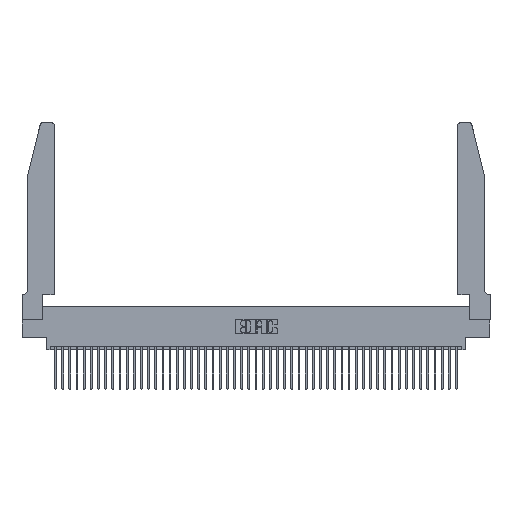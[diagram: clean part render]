
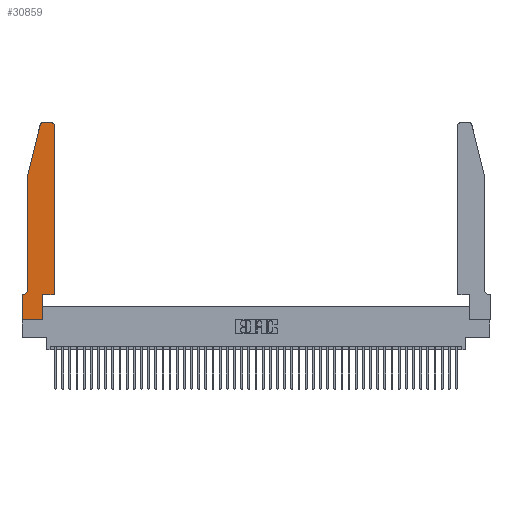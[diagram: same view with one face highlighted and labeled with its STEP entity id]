
A CAD part, top view. The second image highlights one B-rep face of the part: STEP entity #30859.
In plain terms, the highlighted planar face has unit normal (0, 0, 1).
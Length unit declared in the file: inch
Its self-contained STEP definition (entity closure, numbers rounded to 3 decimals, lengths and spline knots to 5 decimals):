
#106 = DIRECTION ( 'NONE',  ( -0.239, -0.971, 0. ) ) ;
#326 = PLANE ( 'NONE',  #36284 ) ;
#693 = LINE ( 'NONE', #32743, #38862 ) ;
#1803 = CARTESIAN_POINT ( 'NONE',  ( 0.0755, 0.42, 0.37 ) ) ;
#2309 = ORIENTED_EDGE ( 'NONE', *, *, #7691, .T. ) ;
#3021 = DIRECTION ( 'NONE',  ( 1., 0., 0. ) ) ;
#4011 = EDGE_CURVE ( 'NONE', #29170, #10294, #20883, .T. ) ;
#4513 = AXIS2_PLACEMENT_3D ( 'NONE', #14572, #40284, #18308 ) ;
#4739 = VERTEX_POINT ( 'NONE', #24880 ) ;
#4830 = EDGE_CURVE ( 'NONE', #10294, #25351, #20247, .T. ) ;
#5912 = VERTEX_POINT ( 'NONE', #9703 ) ;
#6037 = CARTESIAN_POINT ( 'NONE',  ( 0., 0., 0.37 ) ) ;
#6311 = VERTEX_POINT ( 'NONE', #16359 ) ;
#6800 = EDGE_CURVE ( 'NONE', #5912, #36614, #37261, .T. ) ;
#7691 = EDGE_CURVE ( 'NONE', #46700, #10394, #33453, .T. ) ;
#7784 = DIRECTION ( 'NONE',  ( 0., 0., 1. ) ) ;
#8949 = VECTOR ( 'NONE', #31866, 39.37008 ) ;
#9164 = EDGE_CURVE ( 'NONE', #25351, #6311, #40741, .T. ) ;
#9679 = ORIENTED_EDGE ( 'NONE', *, *, #36861, .T. ) ;
#9703 = CARTESIAN_POINT ( 'NONE',  ( 0., 0.35, 0.37 ) ) ;
#9863 = DIRECTION ( 'NONE',  ( 1., 0., 0. ) ) ;
#10294 = VERTEX_POINT ( 'NONE', #19686 ) ;
#10343 = CARTESIAN_POINT ( 'NONE',  ( 0.0755, 0.35, 0.37 ) ) ;
#10394 = VERTEX_POINT ( 'NONE', #12528 ) ;
#10613 = CARTESIAN_POINT ( 'NONE',  ( 0.2865, 0.35, 0.37 ) ) ;
#11379 = VECTOR ( 'NONE', #12833, 39.37008 ) ;
#12073 = VECTOR ( 'NONE', #32721, 39.37008 ) ;
#12437 = VECTOR ( 'NONE', #9863, 39.37008 ) ;
#12528 = CARTESIAN_POINT ( 'NONE',  ( 0.0755, 2., 0.37 ) ) ;
#12833 = DIRECTION ( 'NONE',  ( -1., 0., 0. ) ) ;
#12932 = AXIS2_PLACEMENT_3D ( 'NONE', #40103, #18118, #43701 ) ;
#13871 = ORIENTED_EDGE ( 'NONE', *, *, #18072, .T. ) ;
#14120 = DIRECTION ( 'NONE',  ( -1., 0., 0. ) ) ;
#14572 = CARTESIAN_POINT ( 'NONE',  ( 0.0055, 0.42, 0.37 ) ) ;
#14804 = CARTESIAN_POINT ( 'NONE',  ( 0.4505, 0.35, 0.37 ) ) ;
#16359 = CARTESIAN_POINT ( 'NONE',  ( 0.284, 2.75, 0.37 ) ) ;
#16466 = ORIENTED_EDGE ( 'NONE', *, *, #4830, .T. ) ;
#17728 = VECTOR ( 'NONE', #14120, 39.37008 ) ;
#18072 = EDGE_CURVE ( 'NONE', #18922, #29108, #40275, .T. ) ;
#18118 = DIRECTION ( 'NONE',  ( 0., 0., 1. ) ) ;
#18139 = DIRECTION ( 'NONE',  ( 0., -1., 0. ) ) ;
#18308 = DIRECTION ( 'NONE',  ( -1., 0., 0. ) ) ;
#18481 = ORIENTED_EDGE ( 'NONE', *, *, #43101, .T. ) ;
#18615 = VECTOR ( 'NONE', #3021, 39.37008 ) ;
#18922 = VERTEX_POINT ( 'NONE', #33369 ) ;
#19596 = CARTESIAN_POINT ( 'NONE',  ( 0.284, 2.72, 0.37 ) ) ;
#19686 = CARTESIAN_POINT ( 'NONE',  ( 0.4505, 2.72, 0.37 ) ) ;
#20041 = ORIENTED_EDGE ( 'NONE', *, *, #21690, .T. ) ;
#20247 = CIRCLE ( 'NONE', #12932, 0.03 ) ;
#20604 = CARTESIAN_POINT ( 'NONE',  ( 0.25487, 2.72718, 0.37 ) ) ;
#20883 = LINE ( 'NONE', #20950, #39261 ) ;
#20950 = CARTESIAN_POINT ( 'NONE',  ( 0.4505, 0.35, 0.37 ) ) ;
#21690 = EDGE_CURVE ( 'NONE', #36614, #18922, #23450, .T. ) ;
#22193 = CARTESIAN_POINT ( 'NONE',  ( 0.0755, 2., 0.37 ) ) ;
#22351 = FACE_OUTER_BOUND ( 'NONE', #24355, .T. ) ;
#22957 = ORIENTED_EDGE ( 'NONE', *, *, #46926, .T. ) ;
#23303 = DIRECTION ( 'NONE',  ( 1., 0., 0. ) ) ;
#23450 = LINE ( 'NONE', #28476, #12437 ) ;
#23678 = ORIENTED_EDGE ( 'NONE', *, *, #31571, .T. ) ;
#23704 = VECTOR ( 'NONE', #106, 39.37008 ) ;
#24355 = EDGE_LOOP ( 'NONE', ( #29853, #23678, #2309, #9679, #22957, #18481, #30250, #20041, #13871, #29082, #36806, #16466 ) ) ;
#24656 = CIRCLE ( 'NONE', #4513, 0.07 ) ;
#24880 = CARTESIAN_POINT ( 'NONE',  ( 0.0055, 0.35, 0.37 ) ) ;
#25211 = CARTESIAN_POINT ( 'NONE',  ( 0.4505, 0.35, 0.37 ) ) ;
#25351 = VERTEX_POINT ( 'NONE', #31988 ) ;
#28324 = DIRECTION ( 'NONE',  ( 0., 1., 0. ) ) ;
#28476 = CARTESIAN_POINT ( 'NONE',  ( 0., 0., 0.37 ) ) ;
#29082 = ORIENTED_EDGE ( 'NONE', *, *, #40509, .T. ) ;
#29108 = VERTEX_POINT ( 'NONE', #32825 ) ;
#29170 = VERTEX_POINT ( 'NONE', #14804 ) ;
#29853 = ORIENTED_EDGE ( 'NONE', *, *, #9164, .T. ) ;
#29937 = CARTESIAN_POINT ( 'NONE',  ( 0., 0.35, 0.37 ) ) ;
#30250 = ORIENTED_EDGE ( 'NONE', *, *, #6800, .T. ) ;
#30859 = ADVANCED_FACE ( 'NONE', ( #22351 ), #326, .T. ) ;
#31190 = CARTESIAN_POINT ( 'NONE',  ( 0.2605, 2.75, 0.37 ) ) ;
#31571 = EDGE_CURVE ( 'NONE', #6311, #46700, #41159, .T. ) ;
#31866 = DIRECTION ( 'NONE',  ( 0., -1., 0. ) ) ;
#31988 = CARTESIAN_POINT ( 'NONE',  ( 0.4205, 2.75, 0.37 ) ) ;
#32721 = DIRECTION ( 'NONE',  ( 0., 1., 0. ) ) ;
#32743 = CARTESIAN_POINT ( 'NONE',  ( 0.0755, 2., 0.37 ) ) ;
#32825 = CARTESIAN_POINT ( 'NONE',  ( 0.2865, 0.35, 0.37 ) ) ;
#33369 = CARTESIAN_POINT ( 'NONE',  ( 0.2865, 0., 0.37 ) ) ;
#33453 = LINE ( 'NONE', #22193, #23704 ) ;
#33617 = DIRECTION ( 'NONE',  ( 1., 0., 0. ) ) ;
#36284 = AXIS2_PLACEMENT_3D ( 'NONE', #29937, #7784, #33617 ) ;
#36614 = VERTEX_POINT ( 'NONE', #41658 ) ;
#36806 = ORIENTED_EDGE ( 'NONE', *, *, #4011, .T. ) ;
#36861 = EDGE_CURVE ( 'NONE', #10394, #46107, #693, .T. ) ;
#37261 = LINE ( 'NONE', #6037, #8949 ) ;
#37311 = LINE ( 'NONE', #10343, #17728 ) ;
#38862 = VECTOR ( 'NONE', #18139, 39.37008 ) ;
#39261 = VECTOR ( 'NONE', #28324, 39.37008 ) ;
#40103 = CARTESIAN_POINT ( 'NONE',  ( 0.4205, 2.72, 0.37 ) ) ;
#40275 = LINE ( 'NONE', #10613, #12073 ) ;
#40284 = DIRECTION ( 'NONE',  ( 0., 0., -1. ) ) ;
#40509 = EDGE_CURVE ( 'NONE', #29108, #29170, #46638, .T. ) ;
#40741 = LINE ( 'NONE', #31190, #11379 ) ;
#41159 = CIRCLE ( 'NONE', #44173, 0.03 ) ;
#41658 = CARTESIAN_POINT ( 'NONE',  ( 0., 0., 0.37 ) ) ;
#43101 = EDGE_CURVE ( 'NONE', #4739, #5912, #37311, .T. ) ;
#43701 = DIRECTION ( 'NONE',  ( 1., 0., 0. ) ) ;
#44173 = AXIS2_PLACEMENT_3D ( 'NONE', #19596, #45167, #23303 ) ;
#45167 = DIRECTION ( 'NONE',  ( 0., 0., 1. ) ) ;
#46107 = VERTEX_POINT ( 'NONE', #1803 ) ;
#46638 = LINE ( 'NONE', #25211, #18615 ) ;
#46700 = VERTEX_POINT ( 'NONE', #20604 ) ;
#46926 = EDGE_CURVE ( 'NONE', #46107, #4739, #24656, .T. ) ;
